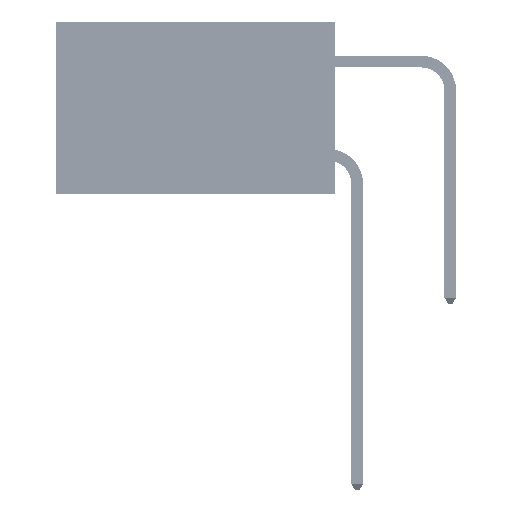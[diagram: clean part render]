
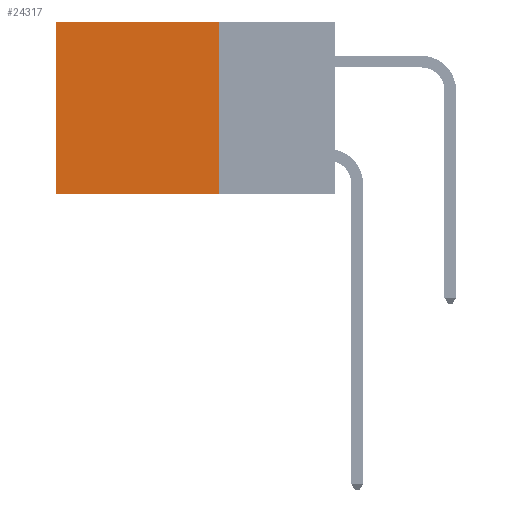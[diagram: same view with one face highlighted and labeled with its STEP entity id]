
A CAD part, left-side view. The second image highlights one B-rep face of the part: STEP entity #24317.
In plain terms, the highlighted planar face has unit normal (-1, 0, 0).
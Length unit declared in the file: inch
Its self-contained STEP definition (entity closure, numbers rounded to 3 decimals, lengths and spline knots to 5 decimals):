
#1028 = ORIENTED_EDGE ( 'NONE', *, *, #53650, .F. ) ;
#2068 = DIRECTION ( 'NONE',  ( 0., 1., 0. ) ) ;
#2452 = CARTESIAN_POINT ( 'NONE',  ( 0.2875, 0.6, 0. ) ) ;
#3150 = ORIENTED_EDGE ( 'NONE', *, *, #43881, .T. ) ;
#4649 = CARTESIAN_POINT ( 'NONE',  ( 0.2875, 0.6, -0.37 ) ) ;
#7039 = VERTEX_POINT ( 'NONE', #39514 ) ;
#8105 = VERTEX_POINT ( 'NONE', #4649 ) ;
#9118 = FACE_OUTER_BOUND ( 'NONE', #48985, .T. ) ;
#13260 = CARTESIAN_POINT ( 'NONE',  ( 0.2875, 0.6, 0. ) ) ;
#13534 = VECTOR ( 'NONE', #30473, 39.37008 ) ;
#18343 = EDGE_CURVE ( 'NONE', #7039, #25827, #52307, .T. ) ;
#18694 = DIRECTION ( 'NONE',  ( 0., 0., -1. ) ) ;
#24317 = ADVANCED_FACE ( 'NONE', ( #9118 ), #35622, .F. ) ;
#24570 = ORIENTED_EDGE ( 'NONE', *, *, #27313, .F. ) ;
#24982 = LINE ( 'NONE', #13260, #13534 ) ;
#25827 = VERTEX_POINT ( 'NONE', #2452 ) ;
#27313 = EDGE_CURVE ( 'NONE', #43146, #8105, #52488, .T. ) ;
#29735 = CARTESIAN_POINT ( 'NONE',  ( 0.2875, 0.25, -0.37 ) ) ;
#29794 = VECTOR ( 'NONE', #2068, 39.37008 ) ;
#30473 = DIRECTION ( 'NONE',  ( 0., 0., -1. ) ) ;
#32147 = CARTESIAN_POINT ( 'NONE',  ( 0.2875, 0.25, 0. ) ) ;
#35622 = PLANE ( 'NONE',  #36342 ) ;
#36342 = AXIS2_PLACEMENT_3D ( 'NONE', #39697, #44207, #18694 ) ;
#39514 = CARTESIAN_POINT ( 'NONE',  ( 0.2875, 0.25, 0. ) ) ;
#39697 = CARTESIAN_POINT ( 'NONE',  ( 0.2875, 0.25, 0. ) ) ;
#42252 = CARTESIAN_POINT ( 'NONE',  ( 0.2875, 0.25, -0.37 ) ) ;
#42611 = VECTOR ( 'NONE', #55066, 39.37008 ) ;
#43146 = VERTEX_POINT ( 'NONE', #42252 ) ;
#43631 = CARTESIAN_POINT ( 'NONE',  ( 0.2875, 0.25, 0. ) ) ;
#43881 = EDGE_CURVE ( 'NONE', #25827, #8105, #24982, .T. ) ;
#44207 = DIRECTION ( 'NONE',  ( 1., 0., 0. ) ) ;
#47518 = VECTOR ( 'NONE', #52085, 39.37008 ) ;
#48834 = LINE ( 'NONE', #43631, #47518 ) ;
#48985 = EDGE_LOOP ( 'NONE', ( #3150, #24570, #1028, #55085 ) ) ;
#52085 = DIRECTION ( 'NONE',  ( 0., 0., -1. ) ) ;
#52307 = LINE ( 'NONE', #32147, #29794 ) ;
#52488 = LINE ( 'NONE', #29735, #42611 ) ;
#53650 = EDGE_CURVE ( 'NONE', #7039, #43146, #48834, .T. ) ;
#55066 = DIRECTION ( 'NONE',  ( 0., 1., 0. ) ) ;
#55085 = ORIENTED_EDGE ( 'NONE', *, *, #18343, .T. ) ;
